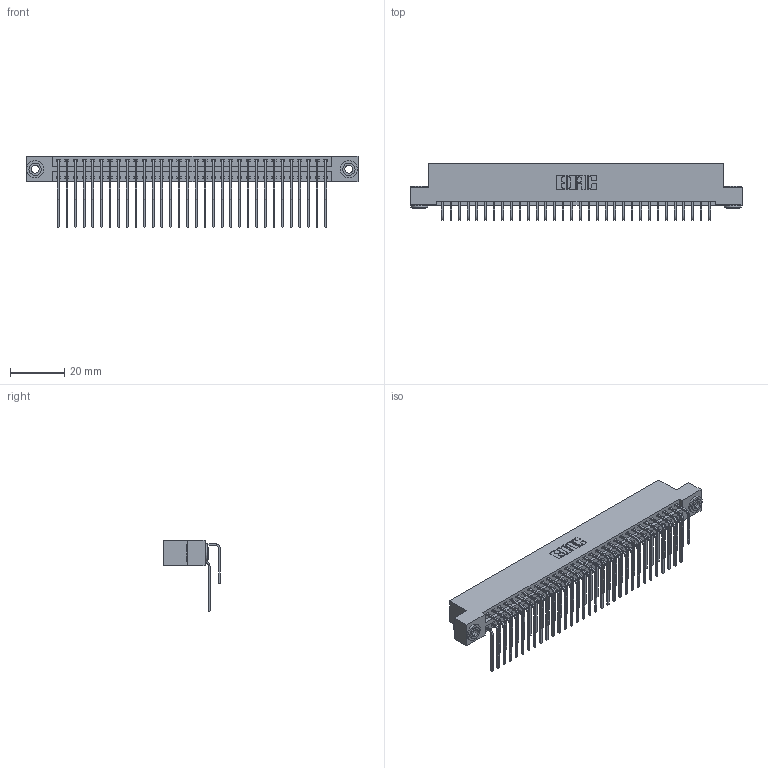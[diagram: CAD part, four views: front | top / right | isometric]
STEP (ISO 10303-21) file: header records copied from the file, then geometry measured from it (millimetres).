
FILE_DESCRIPTION (( 'STEP AP203' ), '1' );
FILE_NAME ('396-064-559-203.STEP', '2018-09-08T18:02:01', ( '' ), ( '' ), 'SwSTEP 2.0', 'SolidWorks 2016', '' );
FILE_SCHEMA (( 'CONFIG_CONTROL_DESIGN' ));
Length unit declared in the file: inch
Products named in the file (5): 346 Part_Flush Mounting Lugs - 0.156 Dia-TH; 345-292-001_558 559 Tail - 1; 345-292-001_559 Tail - 2; 345-250-002_345-250-002-102; 396-064-559-203
Assembly tree (67 placements, depth 2):
  396-064-559-203
    346 Part_Flush Mounting Lugs - 0.156 Dia-TH
    345-292-001_558 559 Tail - 1  x32
    345-292-001_559 Tail - 2  x32
    345-250-002_345-250-002-102  x2
Bounding box: 122.17 x 20.89 x 26.16 mm (x, y, z)
Volume: 12224.4 mm3; surface area: 18631.5 mm2
Topology: 67 solids, 67 shells, 3616 faces, 10709 edges, 7050 vertices
Faces by surface type: plane 2454, cylinder 1154, cone 8
Entity records: 24664 total; most frequent: CARTESIAN_POINT 4106, ORIENTED_EDGE 3982, DIRECTION 3673, EDGE_CURVE 1991, VECTOR 1667, LINE 1667, VERTEX_POINT 1322, AXIS2_PLACEMENT_3D 1003
